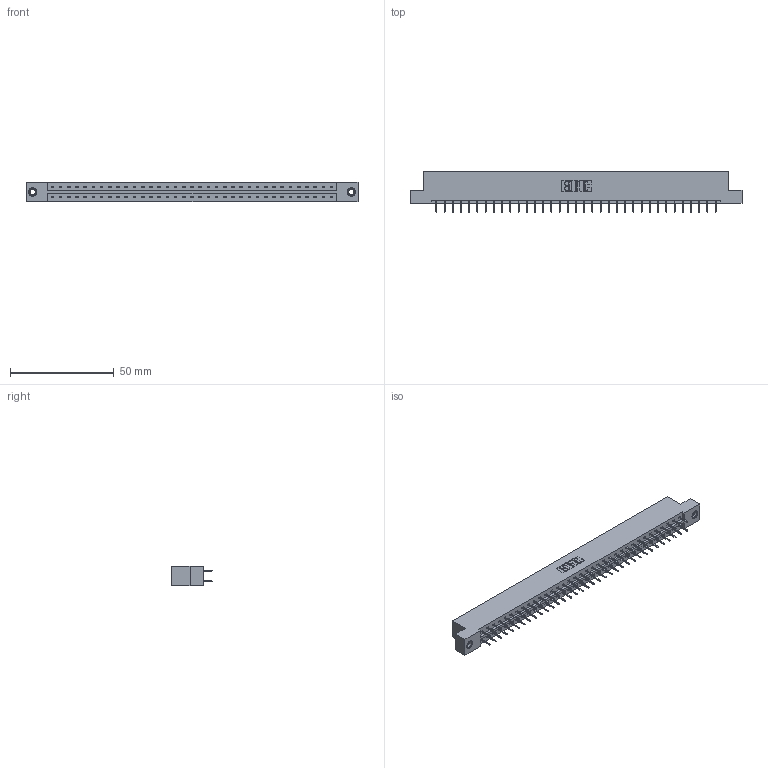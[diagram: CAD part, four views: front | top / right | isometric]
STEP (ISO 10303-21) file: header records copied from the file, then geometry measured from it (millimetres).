
FILE_DESCRIPTION (( 'STEP AP203' ), '1' );
FILE_NAME ('333-070-524-207.STEP', '2018-08-04T14:34:54', ( '' ), ( '' ), 'SwSTEP 2.0', 'SolidWorks 2016', '' );
FILE_SCHEMA (( 'CONFIG_CONTROL_DESIGN' ));
Length unit declared in the file: inch
Products named in the file (4): 345-292-001_345-293-124; 345-250-001_345-250-005-103; 333-070-524-207; 333 Part_Flush - .156 Dia - TI
Assembly tree (73 placements, depth 2):
  333-070-524-207
    333 Part_Flush - .156 Dia - TI
    345-292-001_345-293-124  x70
    345-250-001_345-250-005-103  x2
Bounding box: 160.22 x 19.69 x 9.4 mm (x, y, z)
Volume: 16173 mm3; surface area: 18761.4 mm2
Topology: 73 solids, 73 shells, 4094 faces, 11577 edges, 7430 vertices
Faces by surface type: plane 3042, cylinder 1036, cone 12, torus 4
Entity records: 24682 total; most frequent: CARTESIAN_POINT 4081, ORIENTED_EDGE 4010, DIRECTION 3531, EDGE_CURVE 2005, LINE 1861, VECTOR 1861, VERTEX_POINT 1328, AXIS2_PLACEMENT_3D 835
